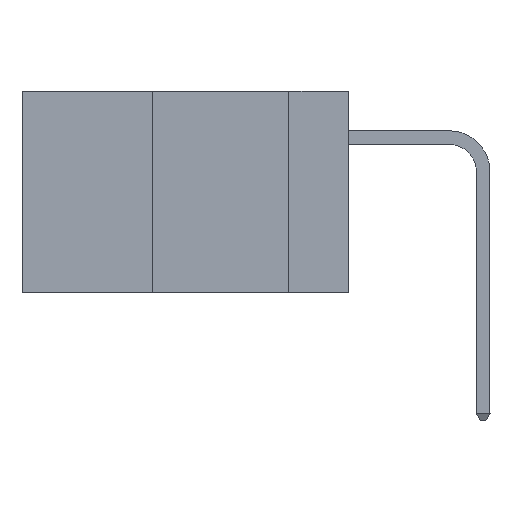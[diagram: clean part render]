
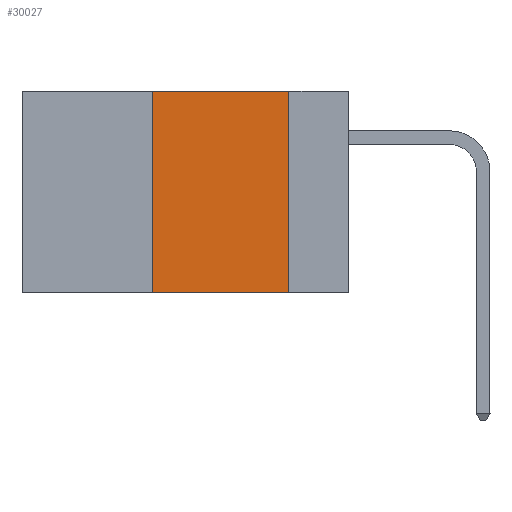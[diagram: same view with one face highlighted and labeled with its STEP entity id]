
A CAD part, left-side view. The second image highlights one B-rep face of the part: STEP entity #30027.
In plain terms, the highlighted planar face has unit normal (-1, 0, 0).
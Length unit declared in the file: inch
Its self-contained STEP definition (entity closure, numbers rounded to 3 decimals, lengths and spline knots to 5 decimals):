
#559 = CARTESIAN_POINT ( 'NONE',  ( 0., 0.36, 0. ) ) ;
#1975 = EDGE_CURVE ( 'NONE', #5492, #37069, #39999, .T. ) ;
#2695 = VECTOR ( 'NONE', #9124, 39.37008 ) ;
#5008 = FACE_OUTER_BOUND ( 'NONE', #13611, .T. ) ;
#5492 = VERTEX_POINT ( 'NONE', #17593 ) ;
#5575 = LINE ( 'NONE', #15368, #34302 ) ;
#8239 = ORIENTED_EDGE ( 'NONE', *, *, #20887, .F. ) ;
#9124 = DIRECTION ( 'NONE',  ( 0., -1., 0. ) ) ;
#13102 = LINE ( 'NONE', #26109, #40124 ) ;
#13611 = EDGE_LOOP ( 'NONE', ( #39370, #8239, #28845, #36436 ) ) ;
#15216 = EDGE_CURVE ( 'NONE', #5492, #31336, #5575, .T. ) ;
#15368 = CARTESIAN_POINT ( 'NONE',  ( 0., 0.6, -0.37 ) ) ;
#16645 = AXIS2_PLACEMENT_3D ( 'NONE', #24409, #37007, #17792 ) ;
#17593 = CARTESIAN_POINT ( 'NONE',  ( 0., 0.36, -0.37 ) ) ;
#17792 = DIRECTION ( 'NONE',  ( 0., 0., -1. ) ) ;
#20782 = PLANE ( 'NONE',  #16645 ) ;
#20887 = EDGE_CURVE ( 'NONE', #37069, #27559, #34928, .T. ) ;
#22826 = EDGE_CURVE ( 'NONE', #27559, #31336, #13102, .T. ) ;
#24409 = CARTESIAN_POINT ( 'NONE',  ( 0., 0.6, 0. ) ) ;
#25442 = CARTESIAN_POINT ( 'NONE',  ( 0., 0.36, 0. ) ) ;
#26109 = CARTESIAN_POINT ( 'NONE',  ( 0., 0.11, 0. ) ) ;
#27559 = VERTEX_POINT ( 'NONE', #29063 ) ;
#28513 = CARTESIAN_POINT ( 'NONE',  ( 0., 0.6, 0. ) ) ;
#28845 = ORIENTED_EDGE ( 'NONE', *, *, #1975, .F. ) ;
#29063 = CARTESIAN_POINT ( 'NONE',  ( 0., 0.11, 0. ) ) ;
#30027 = ADVANCED_FACE ( 'NONE', ( #5008 ), #20782, .F. ) ;
#31336 = VERTEX_POINT ( 'NONE', #33428 ) ;
#32920 = DIRECTION ( 'NONE',  ( 0., 0., -1. ) ) ;
#33155 = DIRECTION ( 'NONE',  ( 0., 0., 1. ) ) ;
#33428 = CARTESIAN_POINT ( 'NONE',  ( 0., 0.11, -0.37 ) ) ;
#34302 = VECTOR ( 'NONE', #38000, 39.37008 ) ;
#34928 = LINE ( 'NONE', #28513, #2695 ) ;
#36436 = ORIENTED_EDGE ( 'NONE', *, *, #15216, .T. ) ;
#37007 = DIRECTION ( 'NONE',  ( 1., 0., 0. ) ) ;
#37069 = VERTEX_POINT ( 'NONE', #25442 ) ;
#38000 = DIRECTION ( 'NONE',  ( 0., -1., 0. ) ) ;
#39311 = VECTOR ( 'NONE', #33155, 39.37008 ) ;
#39370 = ORIENTED_EDGE ( 'NONE', *, *, #22826, .F. ) ;
#39999 = LINE ( 'NONE', #559, #39311 ) ;
#40124 = VECTOR ( 'NONE', #32920, 39.37008 ) ;
